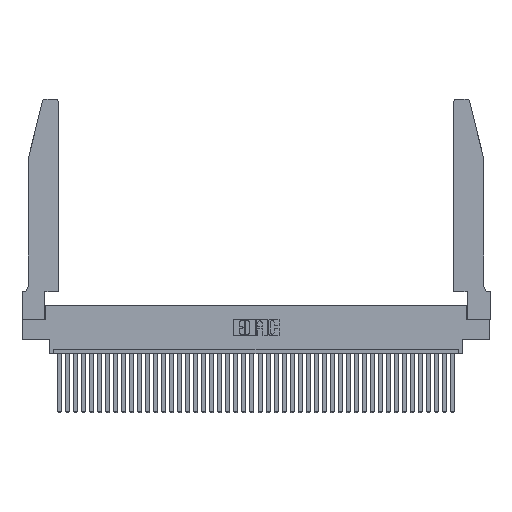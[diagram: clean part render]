
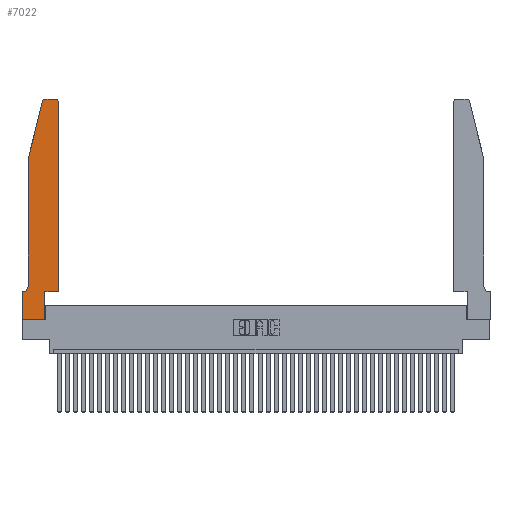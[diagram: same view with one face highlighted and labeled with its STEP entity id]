
A CAD part, top view. The second image highlights one B-rep face of the part: STEP entity #7022.
In plain terms, the highlighted planar face has unit normal (0, 0, 1).
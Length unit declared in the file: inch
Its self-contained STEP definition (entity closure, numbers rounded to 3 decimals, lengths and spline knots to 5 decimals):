
#312 = VECTOR ( 'NONE', #38956, 39.37008 ) ;
#821 = DIRECTION ( 'NONE',  ( -0.239, -0.971, 0. ) ) ;
#1116 = CIRCLE ( 'NONE', #18881, 0.03 ) ;
#1542 = CARTESIAN_POINT ( 'NONE',  ( 0., 0.35, 0.37 ) ) ;
#1557 = CARTESIAN_POINT ( 'NONE',  ( 0.4505, 0.35, 0.37 ) ) ;
#2688 = LINE ( 'NONE', #40164, #27064 ) ;
#2754 = AXIS2_PLACEMENT_3D ( 'NONE', #4733, #7936, #4892 ) ;
#3322 = VERTEX_POINT ( 'NONE', #1557 ) ;
#3841 = CARTESIAN_POINT ( 'NONE',  ( 0.4505, 2.72, 0.37 ) ) ;
#4248 = CARTESIAN_POINT ( 'NONE',  ( 0.0755, 2., 0.37 ) ) ;
#4450 = CIRCLE ( 'NONE', #2754, 0.07 ) ;
#4487 = EDGE_CURVE ( 'NONE', #12949, #30871, #29920, .T. ) ;
#4733 = CARTESIAN_POINT ( 'NONE',  ( 0.0055, 0.42, 0.37 ) ) ;
#4892 = DIRECTION ( 'NONE',  ( -1., 0., 0. ) ) ;
#5090 = VERTEX_POINT ( 'NONE', #26161 ) ;
#5332 = VERTEX_POINT ( 'NONE', #12097 ) ;
#5673 = CARTESIAN_POINT ( 'NONE',  ( 0.0755, 2., 0.37 ) ) ;
#5876 = CARTESIAN_POINT ( 'NONE',  ( 0.2865, 0., 0.37 ) ) ;
#5878 = CARTESIAN_POINT ( 'NONE',  ( 0., 0.35, 0.37 ) ) ;
#5965 = ORIENTED_EDGE ( 'NONE', *, *, #18474, .T. ) ;
#6781 = VECTOR ( 'NONE', #16937, 39.37008 ) ;
#6817 = CARTESIAN_POINT ( 'NONE',  ( 0.4205, 2.72, 0.37 ) ) ;
#7022 = ADVANCED_FACE ( 'NONE', ( #23224 ), #11006, .T. ) ;
#7936 = DIRECTION ( 'NONE',  ( 0., 0., -1. ) ) ;
#8069 = ORIENTED_EDGE ( 'NONE', *, *, #12122, .T. ) ;
#8139 = VECTOR ( 'NONE', #21906, 39.37008 ) ;
#8364 = AXIS2_PLACEMENT_3D ( 'NONE', #1542, #23783, #11156 ) ;
#8699 = DIRECTION ( 'NONE',  ( 1., 0., 0. ) ) ;
#8705 = ORIENTED_EDGE ( 'NONE', *, *, #13503, .T. ) ;
#9885 = CARTESIAN_POINT ( 'NONE',  ( 0.4205, 2.75, 0.37 ) ) ;
#10134 = CARTESIAN_POINT ( 'NONE',  ( 0.0755, 0.35, 0.37 ) ) ;
#10787 = EDGE_CURVE ( 'NONE', #24730, #33065, #38920, .T. ) ;
#10997 = DIRECTION ( 'NONE',  ( 1., 0., 0. ) ) ;
#11006 = PLANE ( 'NONE',  #8364 ) ;
#11156 = DIRECTION ( 'NONE',  ( 1., 0., 0. ) ) ;
#11297 = CARTESIAN_POINT ( 'NONE',  ( 0.284, 2.72, 0.37 ) ) ;
#11368 = ORIENTED_EDGE ( 'NONE', *, *, #21607, .T. ) ;
#11941 = AXIS2_PLACEMENT_3D ( 'NONE', #11297, #40008, #10997 ) ;
#12097 = CARTESIAN_POINT ( 'NONE',  ( 0.2865, 0.35, 0.37 ) ) ;
#12122 = EDGE_CURVE ( 'NONE', #30871, #38359, #2688, .T. ) ;
#12183 = EDGE_CURVE ( 'NONE', #36121, #24730, #31553, .T. ) ;
#12262 = CARTESIAN_POINT ( 'NONE',  ( 0.0755, 0.42, 0.37 ) ) ;
#12949 = VERTEX_POINT ( 'NONE', #5878 ) ;
#13340 = DIRECTION ( 'NONE',  ( 0., 0., 1. ) ) ;
#13503 = EDGE_CURVE ( 'NONE', #36578, #5090, #4450, .T. ) ;
#13549 = EDGE_CURVE ( 'NONE', #33065, #36578, #25843, .T. ) ;
#14105 = CARTESIAN_POINT ( 'NONE',  ( 0.25487, 2.72718, 0.37 ) ) ;
#15715 = ORIENTED_EDGE ( 'NONE', *, *, #21621, .T. ) ;
#16390 = CARTESIAN_POINT ( 'NONE',  ( 0.4505, 0.35, 0.37 ) ) ;
#16532 = LINE ( 'NONE', #22680, #8139 ) ;
#16937 = DIRECTION ( 'NONE',  ( 0., 1., 0. ) ) ;
#18474 = EDGE_CURVE ( 'NONE', #21645, #34365, #1116, .T. ) ;
#18881 = AXIS2_PLACEMENT_3D ( 'NONE', #6817, #13340, #26310 ) ;
#19062 = ORIENTED_EDGE ( 'NONE', *, *, #10787, .T. ) ;
#19263 = EDGE_CURVE ( 'NONE', #5332, #3322, #27519, .T. ) ;
#19270 = EDGE_CURVE ( 'NONE', #38359, #5332, #22951, .T. ) ;
#19744 = CARTESIAN_POINT ( 'NONE',  ( 0.284, 2.75, 0.37 ) ) ;
#21607 = EDGE_CURVE ( 'NONE', #5090, #12949, #26753, .T. ) ;
#21621 = EDGE_CURVE ( 'NONE', #3322, #21645, #23191, .T. ) ;
#21645 = VERTEX_POINT ( 'NONE', #3841 ) ;
#21675 = DIRECTION ( 'NONE',  ( 0., -1., 0. ) ) ;
#21906 = DIRECTION ( 'NONE',  ( -1., 0., 0. ) ) ;
#22680 = CARTESIAN_POINT ( 'NONE',  ( 0.2605, 2.75, 0.37 ) ) ;
#22706 = EDGE_LOOP ( 'NONE', ( #33053, #35381, #19062, #26154, #8705, #11368, #38735, #8069, #29290, #35185, #15715, #5965 ) ) ;
#22951 = LINE ( 'NONE', #33504, #23988 ) ;
#23191 = LINE ( 'NONE', #16390, #6781 ) ;
#23224 = FACE_OUTER_BOUND ( 'NONE', #22706, .T. ) ;
#23696 = DIRECTION ( 'NONE',  ( 0., -1., 0. ) ) ;
#23783 = DIRECTION ( 'NONE',  ( 0., 0., 1. ) ) ;
#23988 = VECTOR ( 'NONE', #39569, 39.37008 ) ;
#24730 = VERTEX_POINT ( 'NONE', #14105 ) ;
#25843 = LINE ( 'NONE', #34529, #37403 ) ;
#26154 = ORIENTED_EDGE ( 'NONE', *, *, #13549, .T. ) ;
#26161 = CARTESIAN_POINT ( 'NONE',  ( 0.0055, 0.35, 0.37 ) ) ;
#26310 = DIRECTION ( 'NONE',  ( 1., 0., 0. ) ) ;
#26753 = LINE ( 'NONE', #10134, #312 ) ;
#27064 = VECTOR ( 'NONE', #8699, 39.37008 ) ;
#27519 = LINE ( 'NONE', #40343, #33511 ) ;
#28796 = CARTESIAN_POINT ( 'NONE',  ( 0., 0., 0.37 ) ) ;
#29290 = ORIENTED_EDGE ( 'NONE', *, *, #19270, .T. ) ;
#29920 = LINE ( 'NONE', #32930, #30991 ) ;
#30871 = VERTEX_POINT ( 'NONE', #28796 ) ;
#30991 = VECTOR ( 'NONE', #23696, 39.37008 ) ;
#31553 = CIRCLE ( 'NONE', #11941, 0.03 ) ;
#32930 = CARTESIAN_POINT ( 'NONE',  ( 0., 0., 0.37 ) ) ;
#33053 = ORIENTED_EDGE ( 'NONE', *, *, #41042, .T. ) ;
#33065 = VERTEX_POINT ( 'NONE', #4248 ) ;
#33504 = CARTESIAN_POINT ( 'NONE',  ( 0.2865, 0.35, 0.37 ) ) ;
#33511 = VECTOR ( 'NONE', #33762, 39.37008 ) ;
#33762 = DIRECTION ( 'NONE',  ( 1., 0., 0. ) ) ;
#34365 = VERTEX_POINT ( 'NONE', #9885 ) ;
#34529 = CARTESIAN_POINT ( 'NONE',  ( 0.0755, 2., 0.37 ) ) ;
#35185 = ORIENTED_EDGE ( 'NONE', *, *, #19263, .T. ) ;
#35381 = ORIENTED_EDGE ( 'NONE', *, *, #12183, .T. ) ;
#36121 = VERTEX_POINT ( 'NONE', #19744 ) ;
#36578 = VERTEX_POINT ( 'NONE', #12262 ) ;
#37403 = VECTOR ( 'NONE', #21675, 39.37008 ) ;
#37934 = VECTOR ( 'NONE', #821, 39.37008 ) ;
#38359 = VERTEX_POINT ( 'NONE', #5876 ) ;
#38735 = ORIENTED_EDGE ( 'NONE', *, *, #4487, .T. ) ;
#38920 = LINE ( 'NONE', #5673, #37934 ) ;
#38956 = DIRECTION ( 'NONE',  ( -1., 0., 0. ) ) ;
#39569 = DIRECTION ( 'NONE',  ( 0., 1., 0. ) ) ;
#40008 = DIRECTION ( 'NONE',  ( 0., 0., 1. ) ) ;
#40164 = CARTESIAN_POINT ( 'NONE',  ( 0., 0., 0.37 ) ) ;
#40343 = CARTESIAN_POINT ( 'NONE',  ( 0.4505, 0.35, 0.37 ) ) ;
#41042 = EDGE_CURVE ( 'NONE', #34365, #36121, #16532, .T. ) ;
